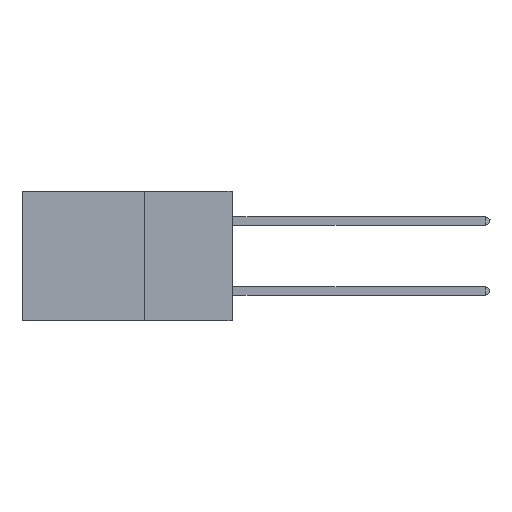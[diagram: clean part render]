
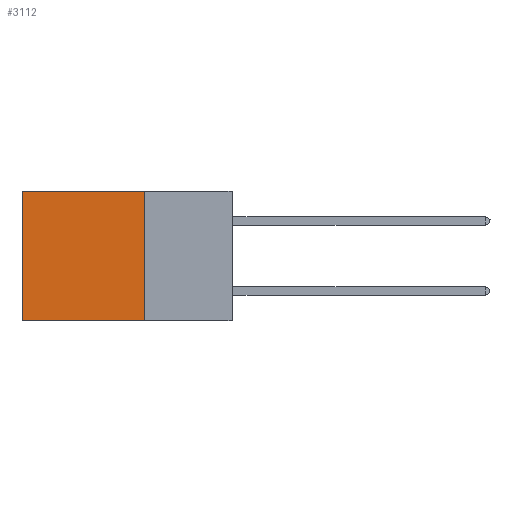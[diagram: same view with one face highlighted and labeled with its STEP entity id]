
A CAD part, left-side view. The second image highlights one B-rep face of the part: STEP entity #3112.
In plain terms, the highlighted planar face has unit normal (-1, 0, 0).
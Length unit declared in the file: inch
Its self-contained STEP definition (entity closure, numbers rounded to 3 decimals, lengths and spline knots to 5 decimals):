
#228 = ORIENTED_EDGE ( 'NONE', *, *, #7551, .T. ) ;
#1496 = CARTESIAN_POINT ( 'NONE',  ( 0.2875, 0.25, -0.37 ) ) ;
#1832 = ORIENTED_EDGE ( 'NONE', *, *, #7850, .F. ) ;
#2625 = VERTEX_POINT ( 'NONE', #9067 ) ;
#2626 = EDGE_CURVE ( 'NONE', #14775, #22677, #5728, .T. ) ;
#2766 = CARTESIAN_POINT ( 'NONE',  ( 0.2875, 0.6, 0. ) ) ;
#3112 = ADVANCED_FACE ( 'NONE', ( #14391 ), #19221, .F. ) ;
#3726 = LINE ( 'NONE', #1496, #22456 ) ;
#5728 = LINE ( 'NONE', #22204, #24926 ) ;
#6342 = DIRECTION ( 'NONE',  ( 0., 0., -1. ) ) ;
#6543 = CARTESIAN_POINT ( 'NONE',  ( 0.2875, 0.25, -0.37 ) ) ;
#6816 = CARTESIAN_POINT ( 'NONE',  ( 0.2875, 0.25, 0. ) ) ;
#7551 = EDGE_CURVE ( 'NONE', #22677, #2625, #21175, .T. ) ;
#7850 = EDGE_CURVE ( 'NONE', #10377, #2625, #3726, .T. ) ;
#8773 = DIRECTION ( 'NONE',  ( 0., 0., -1. ) ) ;
#9067 = CARTESIAN_POINT ( 'NONE',  ( 0.2875, 0.6, -0.37 ) ) ;
#10210 = EDGE_LOOP ( 'NONE', ( #228, #1832, #16961, #25720 ) ) ;
#10377 = VERTEX_POINT ( 'NONE', #6543 ) ;
#11754 = EDGE_CURVE ( 'NONE', #14775, #10377, #23849, .T. ) ;
#14391 = FACE_OUTER_BOUND ( 'NONE', #10210, .T. ) ;
#14775 = VERTEX_POINT ( 'NONE', #15243 ) ;
#14790 = CARTESIAN_POINT ( 'NONE',  ( 0.2875, 0.25, 0. ) ) ;
#15243 = CARTESIAN_POINT ( 'NONE',  ( 0.2875, 0.25, 0. ) ) ;
#16882 = DIRECTION ( 'NONE',  ( 0., 0., -1. ) ) ;
#16961 = ORIENTED_EDGE ( 'NONE', *, *, #11754, .F. ) ;
#18535 = DIRECTION ( 'NONE',  ( 0., 1., 0. ) ) ;
#19221 = PLANE ( 'NONE',  #25332 ) ;
#19397 = VECTOR ( 'NONE', #16882, 39.37008 ) ;
#19983 = DIRECTION ( 'NONE',  ( 0., 1., 0. ) ) ;
#21175 = LINE ( 'NONE', #21310, #19397 ) ;
#21310 = CARTESIAN_POINT ( 'NONE',  ( 0.2875, 0.6, 0. ) ) ;
#22204 = CARTESIAN_POINT ( 'NONE',  ( 0.2875, 0.25, 0. ) ) ;
#22456 = VECTOR ( 'NONE', #18535, 39.37008 ) ;
#22677 = VERTEX_POINT ( 'NONE', #2766 ) ;
#23011 = VECTOR ( 'NONE', #8773, 39.37008 ) ;
#23849 = LINE ( 'NONE', #6816, #23011 ) ;
#24926 = VECTOR ( 'NONE', #19983, 39.37008 ) ;
#25288 = DIRECTION ( 'NONE',  ( 1., 0., 0. ) ) ;
#25332 = AXIS2_PLACEMENT_3D ( 'NONE', #14790, #25288, #6342 ) ;
#25720 = ORIENTED_EDGE ( 'NONE', *, *, #2626, .T. ) ;
